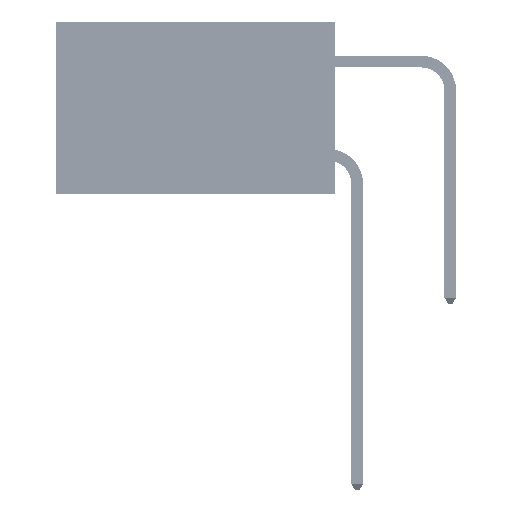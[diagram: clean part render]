
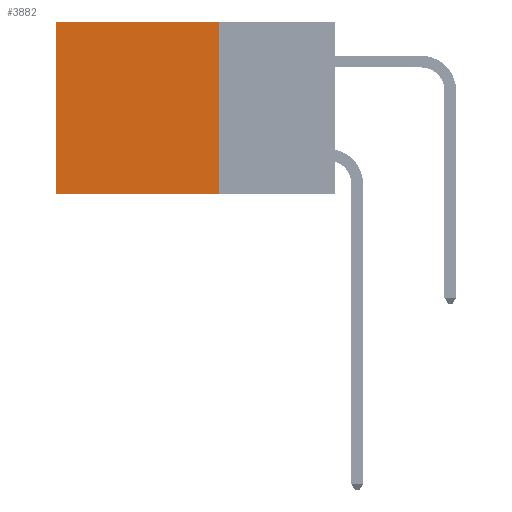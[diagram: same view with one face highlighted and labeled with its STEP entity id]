
A CAD part, left-side view. The second image highlights one B-rep face of the part: STEP entity #3882.
In plain terms, the highlighted planar face has unit normal (-1, 0, 0).
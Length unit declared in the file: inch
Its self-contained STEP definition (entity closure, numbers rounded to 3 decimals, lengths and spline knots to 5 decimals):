
#1046 = VERTEX_POINT ( 'NONE', #45034 ) ;
#2138 = ORIENTED_EDGE ( 'NONE', *, *, #21696, .T. ) ;
#3146 = DIRECTION ( 'NONE',  ( 0., 1., 0. ) ) ;
#3882 = ADVANCED_FACE ( 'NONE', ( #35897 ), #39671, .F. ) ;
#4401 = VERTEX_POINT ( 'NONE', #15119 ) ;
#6305 = ORIENTED_EDGE ( 'NONE', *, *, #17697, .T. ) ;
#8525 = ORIENTED_EDGE ( 'NONE', *, *, #12473, .F. ) ;
#8839 = VERTEX_POINT ( 'NONE', #27567 ) ;
#12473 = EDGE_CURVE ( 'NONE', #4401, #8839, #35168, .T. ) ;
#15119 = CARTESIAN_POINT ( 'NONE',  ( 0.2875, 0.25, -0.37 ) ) ;
#15485 = DIRECTION ( 'NONE',  ( 0., 0., -1. ) ) ;
#16206 = CARTESIAN_POINT ( 'NONE',  ( 0.2875, 0.25, 0. ) ) ;
#17697 = EDGE_CURVE ( 'NONE', #1046, #50589, #45131, .T. ) ;
#20152 = DIRECTION ( 'NONE',  ( 1., 0., 0. ) ) ;
#20889 = DIRECTION ( 'NONE',  ( 0., 1., 0. ) ) ;
#21696 = EDGE_CURVE ( 'NONE', #50589, #8839, #40089, .T. ) ;
#23112 = VECTOR ( 'NONE', #3146, 39.37008 ) ;
#26710 = CARTESIAN_POINT ( 'NONE',  ( 0.2875, 0.25, 0. ) ) ;
#27567 = CARTESIAN_POINT ( 'NONE',  ( 0.2875, 0.6, -0.37 ) ) ;
#29647 = VECTOR ( 'NONE', #15485, 39.37008 ) ;
#32600 = CARTESIAN_POINT ( 'NONE',  ( 0.2875, 0.6, 0. ) ) ;
#33088 = LINE ( 'NONE', #35274, #41060 ) ;
#33696 = EDGE_LOOP ( 'NONE', ( #2138, #8525, #47772, #6305 ) ) ;
#33923 = VECTOR ( 'NONE', #20889, 39.37008 ) ;
#35168 = LINE ( 'NONE', #48256, #33923 ) ;
#35274 = CARTESIAN_POINT ( 'NONE',  ( 0.2875, 0.25, 0. ) ) ;
#35442 = DIRECTION ( 'NONE',  ( 0., 0., -1. ) ) ;
#35897 = FACE_OUTER_BOUND ( 'NONE', #33696, .T. ) ;
#39671 = PLANE ( 'NONE',  #40284 ) ;
#40089 = LINE ( 'NONE', #42722, #29647 ) ;
#40284 = AXIS2_PLACEMENT_3D ( 'NONE', #16206, #20152, #47519 ) ;
#41060 = VECTOR ( 'NONE', #35442, 39.37008 ) ;
#42722 = CARTESIAN_POINT ( 'NONE',  ( 0.2875, 0.6, 0. ) ) ;
#44613 = EDGE_CURVE ( 'NONE', #1046, #4401, #33088, .T. ) ;
#45034 = CARTESIAN_POINT ( 'NONE',  ( 0.2875, 0.25, 0. ) ) ;
#45131 = LINE ( 'NONE', #26710, #23112 ) ;
#47519 = DIRECTION ( 'NONE',  ( 0., 0., -1. ) ) ;
#47772 = ORIENTED_EDGE ( 'NONE', *, *, #44613, .F. ) ;
#48256 = CARTESIAN_POINT ( 'NONE',  ( 0.2875, 0.25, -0.37 ) ) ;
#50589 = VERTEX_POINT ( 'NONE', #32600 ) ;
